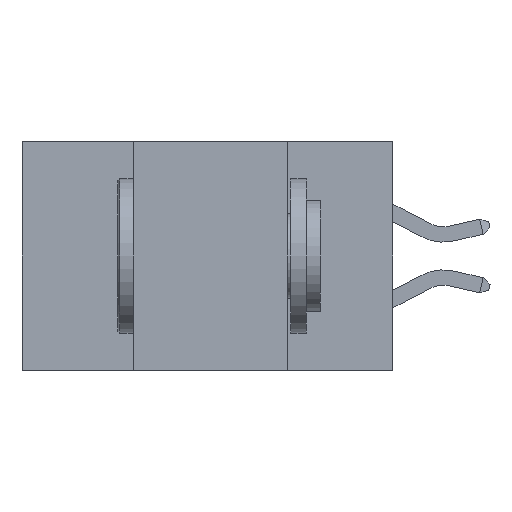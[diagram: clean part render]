
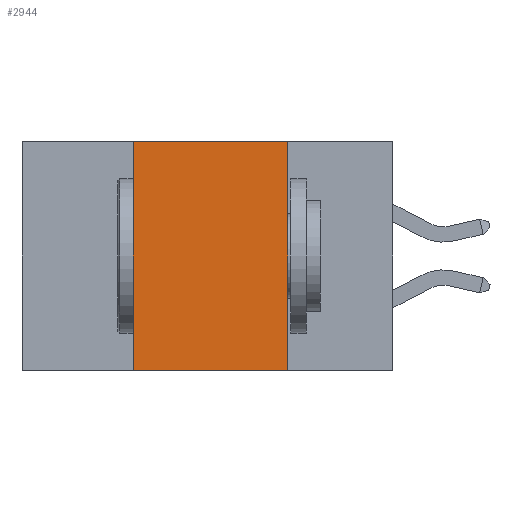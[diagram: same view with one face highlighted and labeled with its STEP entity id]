
A CAD part, left-side view. The second image highlights one B-rep face of the part: STEP entity #2944.
In plain terms, the highlighted planar face has unit normal (-1, 0, 0).
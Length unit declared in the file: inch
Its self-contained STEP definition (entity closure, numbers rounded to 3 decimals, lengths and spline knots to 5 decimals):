
#212 = DIRECTION ( 'NONE',  ( 1., 0., 0. ) ) ;
#586 = CARTESIAN_POINT ( 'NONE',  ( 0., 0.6, 0. ) ) ;
#2944 = ADVANCED_FACE ( 'NONE', ( #26634 ), #35027, .F. ) ;
#6858 = ORIENTED_EDGE ( 'NONE', *, *, #30367, .F. ) ;
#7134 = LINE ( 'NONE', #16933, #37303 ) ;
#7751 = DIRECTION ( 'NONE',  ( 0., 0., -1. ) ) ;
#8437 = CARTESIAN_POINT ( 'NONE',  ( 0., 0.17, -0.37 ) ) ;
#9238 = LINE ( 'NONE', #586, #25270 ) ;
#11423 = ORIENTED_EDGE ( 'NONE', *, *, #13246, .F. ) ;
#12477 = ORIENTED_EDGE ( 'NONE', *, *, #15223, .T. ) ;
#12976 = VERTEX_POINT ( 'NONE', #31427 ) ;
#13246 = EDGE_CURVE ( 'NONE', #14532, #12976, #17066, .T. ) ;
#14532 = VERTEX_POINT ( 'NONE', #36467 ) ;
#14723 = VECTOR ( 'NONE', #24137, 39.37008 ) ;
#14781 = VERTEX_POINT ( 'NONE', #29995 ) ;
#15223 = EDGE_CURVE ( 'NONE', #14532, #37297, #33777, .T. ) ;
#16933 = CARTESIAN_POINT ( 'NONE',  ( 0., 0.17, 0. ) ) ;
#17066 = LINE ( 'NONE', #32735, #14723 ) ;
#17872 = DIRECTION ( 'NONE',  ( 0., 0., -1. ) ) ;
#21455 = ORIENTED_EDGE ( 'NONE', *, *, #22616, .F. ) ;
#22616 = EDGE_CURVE ( 'NONE', #12976, #14781, #9238, .T. ) ;
#23963 = DIRECTION ( 'NONE',  ( 0., -1., 0. ) ) ;
#24137 = DIRECTION ( 'NONE',  ( 0., 0., 1. ) ) ;
#24548 = CARTESIAN_POINT ( 'NONE',  ( 0., 0.6, -0.37 ) ) ;
#25270 = VECTOR ( 'NONE', #23963, 39.37008 ) ;
#26634 = FACE_OUTER_BOUND ( 'NONE', #27018, .T. ) ;
#26762 = AXIS2_PLACEMENT_3D ( 'NONE', #29405, #212, #17872 ) ;
#27018 = EDGE_LOOP ( 'NONE', ( #6858, #21455, #11423, #12477 ) ) ;
#27863 = VECTOR ( 'NONE', #36485, 39.37008 ) ;
#29405 = CARTESIAN_POINT ( 'NONE',  ( 0., 0.6, 0. ) ) ;
#29995 = CARTESIAN_POINT ( 'NONE',  ( 0., 0.17, 0. ) ) ;
#30367 = EDGE_CURVE ( 'NONE', #14781, #37297, #7134, .T. ) ;
#31427 = CARTESIAN_POINT ( 'NONE',  ( 0., 0.42, 0. ) ) ;
#32735 = CARTESIAN_POINT ( 'NONE',  ( 0., 0.42, 0. ) ) ;
#33777 = LINE ( 'NONE', #24548, #27863 ) ;
#35027 = PLANE ( 'NONE',  #26762 ) ;
#36467 = CARTESIAN_POINT ( 'NONE',  ( 0., 0.42, -0.37 ) ) ;
#36485 = DIRECTION ( 'NONE',  ( 0., -1., 0. ) ) ;
#37297 = VERTEX_POINT ( 'NONE', #8437 ) ;
#37303 = VECTOR ( 'NONE', #7751, 39.37008 ) ;
